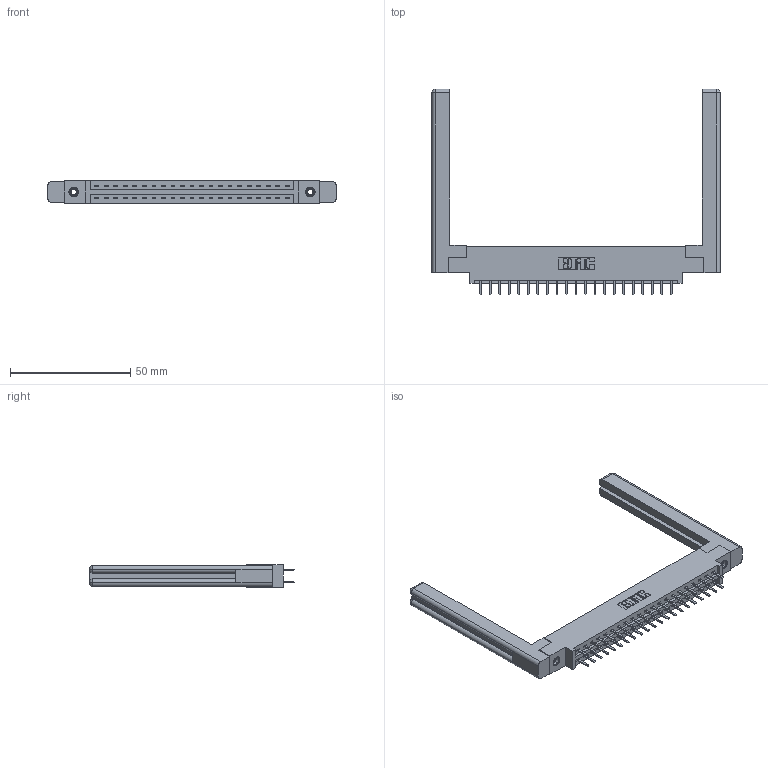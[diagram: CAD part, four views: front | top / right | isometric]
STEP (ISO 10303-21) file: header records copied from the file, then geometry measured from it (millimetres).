
FILE_DESCRIPTION (( 'STEP AP203' ), '1' );
FILE_NAME ('387-042-520-858.STEP', '2019-10-18T03:38:40', ( '' ), ( '' ), 'SwSTEP 2.0', 'SolidWorks 2016', '' );
FILE_SCHEMA (( 'CONFIG_CONTROL_DESIGN' ));
Length unit declared in the file: inch
Products named in the file (5): 307-220-058; 345-250-001_345-250-001-102; 387-042-520-858; 337 Part_0.170 Offset - 0.156 Dia-TI; 345-292-001_345-293-120
Assembly tree (47 placements, depth 2):
  387-042-520-858
    337 Part_0.170 Offset - 0.156 Dia-TI
    345-292-001_345-293-120  x42
    345-250-001_345-250-001-102  x2
    307-220-058  x2
Bounding box: 119.84 x 85.43 x 9.4 mm (x, y, z)
Volume: 19356.2 mm3; surface area: 18705.8 mm2
Topology: 47 solids, 47 shells, 2696 faces, 7775 edges, 5058 vertices
Faces by surface type: plane 1838, cylinder 834, cone 12, torus 12
Entity records: 21878 total; most frequent: CARTESIAN_POINT 3725, ORIENTED_EDGE 3588, DIRECTION 3210, EDGE_CURVE 1794, VECTOR 1614, LINE 1614, VERTEX_POINT 1186, AXIS2_PLACEMENT_3D 798
